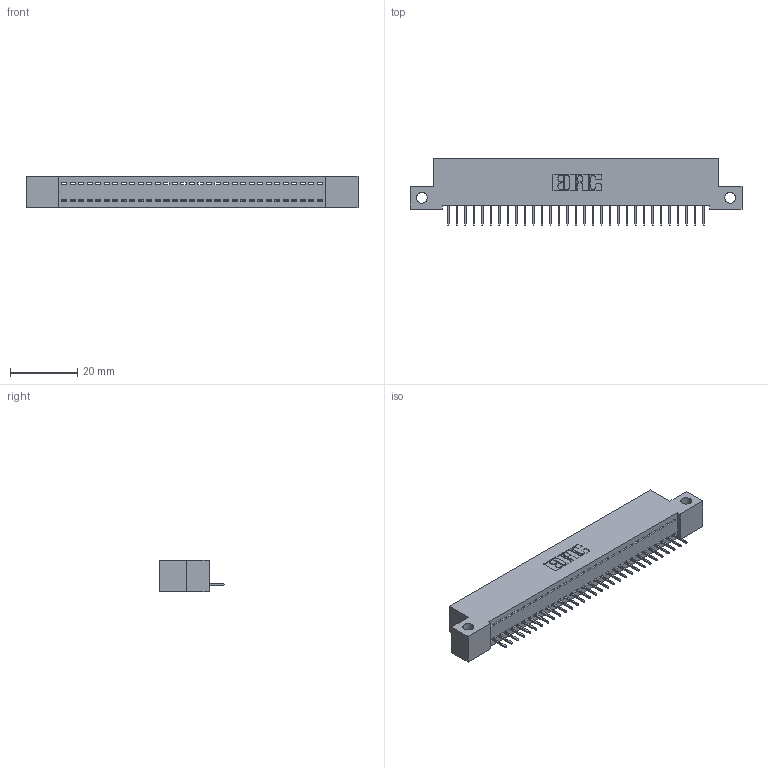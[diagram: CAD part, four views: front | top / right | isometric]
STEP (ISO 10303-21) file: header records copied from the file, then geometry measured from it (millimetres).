
FILE_DESCRIPTION (( 'STEP AP203' ), '1' );
FILE_NAME ('342-031-524-112.STEP', '2019-10-02T05:32:58', ( '' ), ( '' ), 'SwSTEP 2.0', 'SolidWorks 2016', '' );
FILE_SCHEMA (( 'CONFIG_CONTROL_DESIGN' ));
Length unit declared in the file: inch
Products named in the file (3): 342-031-524-112; 342 Part_Side Mount; 345-292-001_345-293-124
Assembly tree (32 placements, depth 2):
  342-031-524-112
    342 Part_Side Mount
    345-292-001_345-293-124  x31
Bounding box: 99.06 x 19.69 x 9.4 mm (x, y, z)
Volume: 8448.7 mm3; surface area: 11657.6 mm2
Topology: 32 solids, 32 shells, 2032 faces, 5879 edges, 3794 vertices
Faces by surface type: plane 1554, cylinder 478
Entity records: 20319 total; most frequent: CARTESIAN_POINT 3511, ORIENTED_EDGE 3478, DIRECTION 2985, EDGE_CURVE 1739, VECTOR 1615, LINE 1615, VERTEX_POINT 1154, AXIS2_PLACEMENT_3D 685
